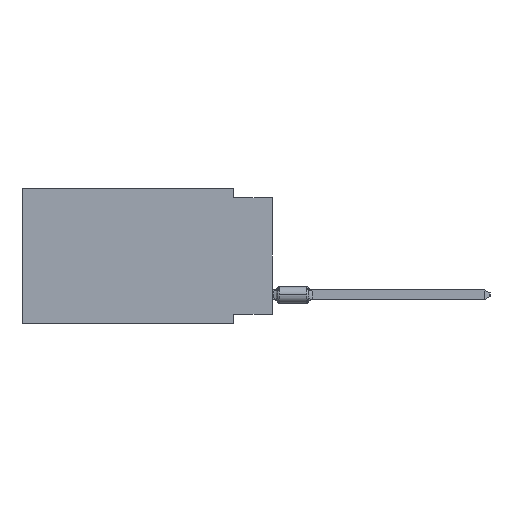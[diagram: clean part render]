
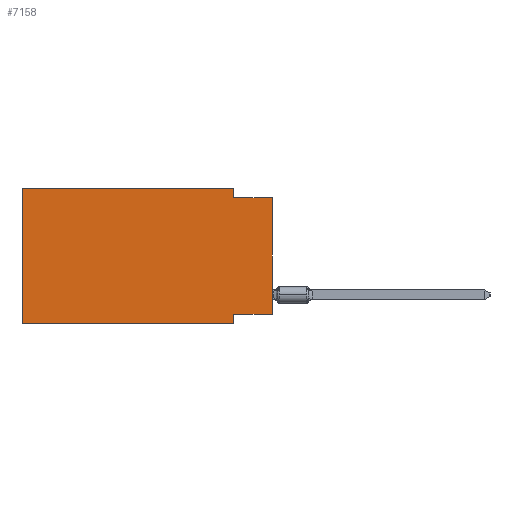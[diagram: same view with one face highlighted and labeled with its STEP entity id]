
A CAD part, left-side view. The second image highlights one B-rep face of the part: STEP entity #7158.
In plain terms, the highlighted planar face has unit normal (-1, 0, 0).
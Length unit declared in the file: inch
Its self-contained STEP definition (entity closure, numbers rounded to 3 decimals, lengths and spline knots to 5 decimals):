
#56 = CARTESIAN_POINT ( 'NONE',  ( 0., 0., -0.025 ) ) ;
#101 = DIRECTION ( 'NONE',  ( 1., 0., 0. ) ) ;
#543 = FACE_OUTER_BOUND ( 'NONE', #1863, .T. ) ;
#1863 = EDGE_LOOP ( 'NONE', ( #31413, #11922, #14238, #31390, #41157, #5448, #7404, #20604 ) ) ;
#2841 = CARTESIAN_POINT ( 'NONE',  ( 0., 0.645, 0. ) ) ;
#3022 = VECTOR ( 'NONE', #23168, 39.37008 ) ;
#5448 = ORIENTED_EDGE ( 'NONE', *, *, #37400, .T. ) ;
#7029 = VECTOR ( 'NONE', #22866, 39.37008 ) ;
#7158 = ADVANCED_FACE ( 'NONE', ( #543 ), #29817, .F. ) ;
#7362 = LINE ( 'NONE', #37271, #29238 ) ;
#7404 = ORIENTED_EDGE ( 'NONE', *, *, #24431, .F. ) ;
#7555 = VERTEX_POINT ( 'NONE', #56 ) ;
#7950 = VECTOR ( 'NONE', #27661, 39.37008 ) ;
#8016 = VERTEX_POINT ( 'NONE', #20593 ) ;
#11922 = ORIENTED_EDGE ( 'NONE', *, *, #38414, .F. ) ;
#13492 = EDGE_CURVE ( 'NONE', #23232, #18393, #16281, .T. ) ;
#13759 = DIRECTION ( 'NONE',  ( 0., 0., -1. ) ) ;
#14169 = CARTESIAN_POINT ( 'NONE',  ( 0., 0.645, -0.35 ) ) ;
#14238 = ORIENTED_EDGE ( 'NONE', *, *, #15423, .F. ) ;
#14390 = CARTESIAN_POINT ( 'NONE',  ( 0., 0.1, -0.35 ) ) ;
#14497 = DIRECTION ( 'NONE',  ( 0., 0., -1. ) ) ;
#15282 = CARTESIAN_POINT ( 'NONE',  ( 0., 0., -0.025 ) ) ;
#15423 = EDGE_CURVE ( 'NONE', #33790, #34456, #36801, .T. ) ;
#16281 = LINE ( 'NONE', #2841, #26952 ) ;
#16321 = CARTESIAN_POINT ( 'NONE',  ( 0., 0.645, 0. ) ) ;
#17540 = VECTOR ( 'NONE', #28428, 39.37008 ) ;
#18393 = VERTEX_POINT ( 'NONE', #35442 ) ;
#19830 = CARTESIAN_POINT ( 'NONE',  ( 0., 0.1, -0.025 ) ) ;
#20593 = CARTESIAN_POINT ( 'NONE',  ( 0., 0.1, -0.325 ) ) ;
#20604 = ORIENTED_EDGE ( 'NONE', *, *, #34078, .F. ) ;
#20657 = VERTEX_POINT ( 'NONE', #25675 ) ;
#21366 = CARTESIAN_POINT ( 'NONE',  ( 0., 0., 0. ) ) ;
#22866 = DIRECTION ( 'NONE',  ( 0., -1., 0. ) ) ;
#23027 = CARTESIAN_POINT ( 'NONE',  ( 0., 0.1, 0. ) ) ;
#23168 = DIRECTION ( 'NONE',  ( 0., 0., -1. ) ) ;
#23232 = VERTEX_POINT ( 'NONE', #34944 ) ;
#23554 = VECTOR ( 'NONE', #28041, 39.37008 ) ;
#24201 = LINE ( 'NONE', #21366, #7950 ) ;
#24431 = EDGE_CURVE ( 'NONE', #8016, #40711, #7362, .T. ) ;
#25179 = LINE ( 'NONE', #31699, #17540 ) ;
#25675 = CARTESIAN_POINT ( 'NONE',  ( 0., 0., -0.325 ) ) ;
#26952 = VECTOR ( 'NONE', #39462, 39.37008 ) ;
#27661 = DIRECTION ( 'NONE',  ( 0., 0., 1. ) ) ;
#28041 = DIRECTION ( 'NONE',  ( 0., -1., 0. ) ) ;
#28428 = DIRECTION ( 'NONE',  ( 0., 1., 0. ) ) ;
#29238 = VECTOR ( 'NONE', #14497, 39.37008 ) ;
#29817 = PLANE ( 'NONE',  #35060 ) ;
#31303 = LINE ( 'NONE', #14169, #23554 ) ;
#31390 = ORIENTED_EDGE ( 'NONE', *, *, #32798, .F. ) ;
#31413 = ORIENTED_EDGE ( 'NONE', *, *, #35716, .T. ) ;
#31699 = CARTESIAN_POINT ( 'NONE',  ( 0., 0., -0.325 ) ) ;
#32638 = LINE ( 'NONE', #15282, #7029 ) ;
#32689 = VECTOR ( 'NONE', #42554, 39.37008 ) ;
#32725 = CARTESIAN_POINT ( 'NONE',  ( 0., 0.1, 0. ) ) ;
#32798 = EDGE_CURVE ( 'NONE', #18393, #33790, #39501, .T. ) ;
#33790 = VERTEX_POINT ( 'NONE', #23027 ) ;
#34078 = EDGE_CURVE ( 'NONE', #20657, #8016, #25179, .T. ) ;
#34456 = VERTEX_POINT ( 'NONE', #19830 ) ;
#34944 = CARTESIAN_POINT ( 'NONE',  ( 0., 0.645, -0.35 ) ) ;
#35060 = AXIS2_PLACEMENT_3D ( 'NONE', #39562, #101, #13759 ) ;
#35442 = CARTESIAN_POINT ( 'NONE',  ( 0., 0.645, 0. ) ) ;
#35716 = EDGE_CURVE ( 'NONE', #20657, #7555, #24201, .T. ) ;
#36801 = LINE ( 'NONE', #32725, #3022 ) ;
#37271 = CARTESIAN_POINT ( 'NONE',  ( 0., 0.1, -0.35 ) ) ;
#37400 = EDGE_CURVE ( 'NONE', #23232, #40711, #31303, .T. ) ;
#38414 = EDGE_CURVE ( 'NONE', #34456, #7555, #32638, .T. ) ;
#39462 = DIRECTION ( 'NONE',  ( 0., 0., 1. ) ) ;
#39501 = LINE ( 'NONE', #16321, #32689 ) ;
#39562 = CARTESIAN_POINT ( 'NONE',  ( 0., 0.645, 0. ) ) ;
#40711 = VERTEX_POINT ( 'NONE', #14390 ) ;
#41157 = ORIENTED_EDGE ( 'NONE', *, *, #13492, .F. ) ;
#42554 = DIRECTION ( 'NONE',  ( 0., -1., 0. ) ) ;
